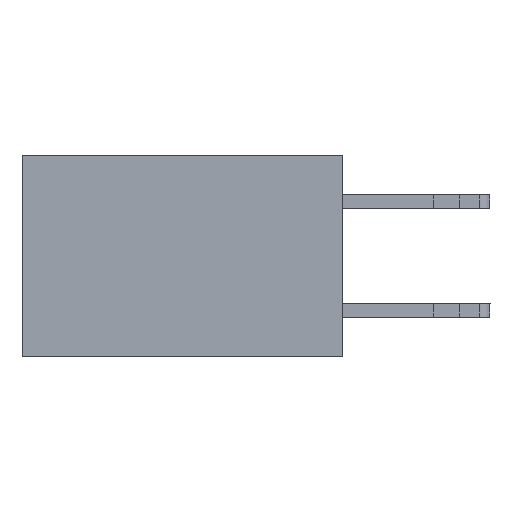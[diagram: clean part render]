
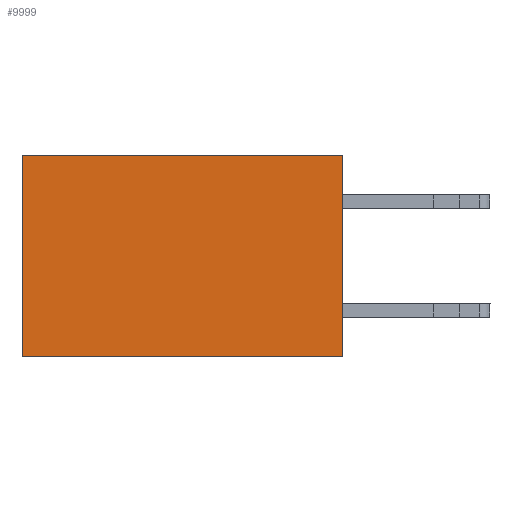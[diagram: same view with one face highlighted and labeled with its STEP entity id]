
A CAD part, left-side view. The second image highlights one B-rep face of the part: STEP entity #9999.
In plain terms, the highlighted planar face has unit normal (-1, 0, 0).
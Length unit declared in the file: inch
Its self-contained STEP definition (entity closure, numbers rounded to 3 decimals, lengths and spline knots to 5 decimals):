
#569 = VERTEX_POINT ( 'NONE', #9347 ) ;
#856 = DIRECTION ( 'NONE',  ( 0., 1., 0. ) ) ;
#861 = DIRECTION ( 'NONE',  ( 0., 1., 0. ) ) ;
#1638 = VECTOR ( 'NONE', #19497, 39.37008 ) ;
#1830 = VECTOR ( 'NONE', #861, 39.37008 ) ;
#2075 = ORIENTED_EDGE ( 'NONE', *, *, #18449, .F. ) ;
#2228 = VECTOR ( 'NONE', #25003, 39.37008 ) ;
#2308 = CARTESIAN_POINT ( 'NONE',  ( 0.277, 0.59, -0.37 ) ) ;
#2591 = PLANE ( 'NONE',  #11665 ) ;
#2661 = CARTESIAN_POINT ( 'NONE',  ( 0.277, 0.59, -0.37 ) ) ;
#2874 = LINE ( 'NONE', #2308, #2228 ) ;
#3005 = VECTOR ( 'NONE', #856, 39.37008 ) ;
#3044 = EDGE_CURVE ( 'NONE', #22476, #14841, #2874, .T. ) ;
#3724 = ORIENTED_EDGE ( 'NONE', *, *, #10813, .T. ) ;
#4780 = CARTESIAN_POINT ( 'NONE',  ( 0.277, 0., -0.37 ) ) ;
#6853 = DIRECTION ( 'NONE',  ( 0., 0., -1. ) ) ;
#7092 = CARTESIAN_POINT ( 'NONE',  ( 0.277, 0., 0. ) ) ;
#7988 = EDGE_LOOP ( 'NONE', ( #12729, #14013, #2075, #3724 ) ) ;
#9347 = CARTESIAN_POINT ( 'NONE',  ( 0.277, 0., 0. ) ) ;
#9999 = ADVANCED_FACE ( 'NONE', ( #21791 ), #2591, .F. ) ;
#10274 = VERTEX_POINT ( 'NONE', #22082 ) ;
#10813 = EDGE_CURVE ( 'NONE', #569, #22476, #24265, .T. ) ;
#11665 = AXIS2_PLACEMENT_3D ( 'NONE', #4780, #19211, #6853 ) ;
#12729 = ORIENTED_EDGE ( 'NONE', *, *, #3044, .T. ) ;
#13285 = CARTESIAN_POINT ( 'NONE',  ( 0.277, 0., -0.37 ) ) ;
#14013 = ORIENTED_EDGE ( 'NONE', *, *, #14897, .F. ) ;
#14841 = VERTEX_POINT ( 'NONE', #2661 ) ;
#14897 = EDGE_CURVE ( 'NONE', #10274, #14841, #18312, .T. ) ;
#18312 = LINE ( 'NONE', #25491, #1830 ) ;
#18449 = EDGE_CURVE ( 'NONE', #569, #10274, #23546, .T. ) ;
#19211 = DIRECTION ( 'NONE',  ( 1., 0., 0. ) ) ;
#19497 = DIRECTION ( 'NONE',  ( 0., 0., -1. ) ) ;
#20793 = CARTESIAN_POINT ( 'NONE',  ( 0.277, 0.59, 0. ) ) ;
#21791 = FACE_OUTER_BOUND ( 'NONE', #7988, .T. ) ;
#22082 = CARTESIAN_POINT ( 'NONE',  ( 0.277, 0., -0.37 ) ) ;
#22476 = VERTEX_POINT ( 'NONE', #20793 ) ;
#23546 = LINE ( 'NONE', #13285, #1638 ) ;
#24265 = LINE ( 'NONE', #7092, #3005 ) ;
#25003 = DIRECTION ( 'NONE',  ( 0., 0., -1. ) ) ;
#25491 = CARTESIAN_POINT ( 'NONE',  ( 0.277, 0., -0.37 ) ) ;
